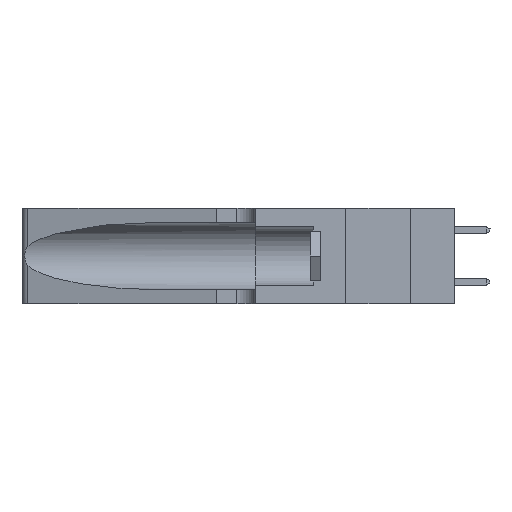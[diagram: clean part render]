
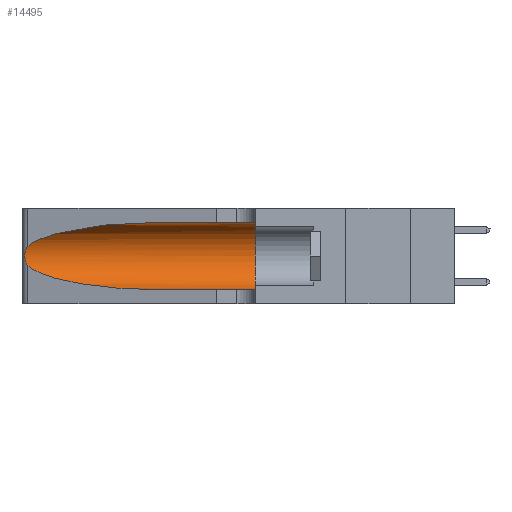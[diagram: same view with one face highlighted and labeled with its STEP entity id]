
A CAD part, left-side view. The second image highlights one B-rep face of the part: STEP entity #14495.
In plain terms, the highlighted cylindrical face has radius 3.308 mm (diameter 6.617 mm), a partial arc.
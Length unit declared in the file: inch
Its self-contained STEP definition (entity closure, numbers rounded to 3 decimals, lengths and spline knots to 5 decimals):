
#180 = ORIENTED_EDGE ( 'NONE', *, *, #1704, .T. ) ;
#356 = VERTEX_POINT ( 'NONE', #25758 ) ;
#576 = CYLINDRICAL_SURFACE ( 'NONE', #26483, 0.13025 ) ;
#1097 = CIRCLE ( 'NONE', #24617, 0.13025 ) ;
#1139 = CARTESIAN_POINT ( 'NONE',  ( 0.1305, 1.61858, 0.05475 ) ) ;
#1341 = FACE_OUTER_BOUND ( 'NONE', #19082, .T. ) ;
#1704 = EDGE_CURVE ( 'NONE', #27995, #356, #4668, .T. ) ;
#2259 = CARTESIAN_POINT ( 'NONE',  ( 0.25487, 1.22718, 0.14631 ) ) ;
#2595 = CARTESIAN_POINT ( 'NONE',  ( 0.25787, 1.23484, 0.2124 ) ) ;
#3226 = VERTEX_POINT ( 'NONE', #3661 ) ;
#3429 = ORIENTED_EDGE ( 'NONE', *, *, #3481, .F. ) ;
#3481 = EDGE_CURVE ( 'NONE', #3226, #27902, #1097, .T. ) ;
#3551 = DIRECTION ( 'NONE',  ( 0., -1., 0. ) ) ;
#3661 = CARTESIAN_POINT ( 'NONE',  ( 0.1305, 0.35, 0.31525 ) ) ;
#4051 = VERTEX_POINT ( 'NONE', #26782 ) ;
#4668 = B_SPLINE_CURVE_WITH_KNOTS ( 'NONE', 3,
 ( #29198, #12241, #17131, #2595, #19552, #5005, #22022, #7479, #24459, #9923, #26884, #12354, #29300, #14800 ),
 .UNSPECIFIED., .F., .F.,
 ( 4, 2, 2, 2, 2, 2, 4 ),
 ( 0., 0.00027, 0.00053, 0.00107, 0.0016, 0.00187, 0.00214 ),
 .UNSPECIFIED. ) ;
#5005 = CARTESIAN_POINT ( 'NONE',  ( 0.26018, 1.23835, 0.19895 ) ) ;
#6705 = CARTESIAN_POINT ( 'NONE',  ( 0.1305, 1.61858, 0.185 ) ) ;
#7057 = DIRECTION ( 'NONE',  ( 0., 1., 0. ) ) ;
#7140 = CARTESIAN_POINT ( 'NONE',  ( 0.1305, 0.72297, 0.05475 ) ) ;
#7352 = CARTESIAN_POINT ( 'NONE',  ( 0.25487, 1.22718, 0.22369 ) ) ;
#7479 = CARTESIAN_POINT ( 'NONE',  ( 0.26075, 1.23896, 0.178 ) ) ;
#7570 = CARTESIAN_POINT ( 'NONE',  ( 0.25487, 1.22718, 0.22369 ) ) ;
#7640 = EDGE_CURVE ( 'NONE', #356, #4051, #24942, .T. ) ;
#8722 = VECTOR ( 'NONE', #3551, 39.37008 ) ;
#9594 = EDGE_CURVE ( 'NONE', #25639, #27995, #13658, .T. ) ;
#9923 = CARTESIAN_POINT ( 'NONE',  ( 0.25856, 1.23593, 0.16098 ) ) ;
#11594 = DIRECTION ( 'NONE',  ( 0., 0., -1. ) ) ;
#12125 = CARTESIAN_POINT ( 'NONE',  ( 0.1305, 0.72297, 0.31525 ) ) ;
#12241 = CARTESIAN_POINT ( 'NONE',  ( 0.25555, 1.22994, 0.2215 ) ) ;
#12354 = CARTESIAN_POINT ( 'NONE',  ( 0.25639, 1.23186, 0.15144 ) ) ;
#12795 = ORIENTED_EDGE ( 'NONE', *, *, #19862, .F. ) ;
#13658 =( BOUNDED_CURVE ( )  B_SPLINE_CURVE ( 3, ( #12125, #19435, #21902, #7352 ),
 .UNSPECIFIED., .F., .F. ) 
 B_SPLINE_CURVE_WITH_KNOTS ( ( 4, 4 ),
 ( 1.5708, 2.84003 ),
 .UNSPECIFIED. ) 
 CURVE ( )  GEOMETRIC_REPRESENTATION_ITEM ( )  RATIONAL_B_SPLINE_CURVE ( ( 1., 0.87, 0.87, 1. ) ) 
 REPRESENTATION_ITEM ( '' )  );
#14286 = ORIENTED_EDGE ( 'NONE', *, *, #7640, .T. ) ;
#14410 = DIRECTION ( 'NONE',  ( 0., -1., 0. ) ) ;
#14495 = ADVANCED_FACE ( 'NONE', ( #1341 ), #576, .F. ) ;
#14800 = CARTESIAN_POINT ( 'NONE',  ( 0.25487, 1.22718, 0.14631 ) ) ;
#16094 = CARTESIAN_POINT ( 'NONE',  ( 0.1305, 0.72297, 0.31525 ) ) ;
#16589 = VECTOR ( 'NONE', #14410, 39.37008 ) ;
#17131 = CARTESIAN_POINT ( 'NONE',  ( 0.25639, 1.23184, 0.21858 ) ) ;
#19082 = EDGE_LOOP ( 'NONE', ( #22947, #180, #14286, #27629, #3429, #12795 ) ) ;
#19220 = CARTESIAN_POINT ( 'NONE',  ( 0.2373, 1.15595, 0.08982 ) ) ;
#19435 = CARTESIAN_POINT ( 'NONE',  ( 0.18966, 0.96281, 0.31525 ) ) ;
#19552 = CARTESIAN_POINT ( 'NONE',  ( 0.25854, 1.2359, 0.20912 ) ) ;
#19862 = EDGE_CURVE ( 'NONE', #25639, #3226, #23037, .T. ) ;
#21618 = CARTESIAN_POINT ( 'NONE',  ( 0.1305, 0.35, 0.185 ) ) ;
#21632 = LINE ( 'NONE', #1139, #8722 ) ;
#21636 = CARTESIAN_POINT ( 'NONE',  ( 0.1305, 1.61858, 0.31525 ) ) ;
#21693 = CARTESIAN_POINT ( 'NONE',  ( 0.18966, 0.96281, 0.05475 ) ) ;
#21902 = CARTESIAN_POINT ( 'NONE',  ( 0.2373, 1.15595, 0.28018 ) ) ;
#22022 = CARTESIAN_POINT ( 'NONE',  ( 0.26075, 1.23896, 0.19203 ) ) ;
#22947 = ORIENTED_EDGE ( 'NONE', *, *, #9594, .T. ) ;
#23037 = LINE ( 'NONE', #21636, #16589 ) ;
#23704 = DIRECTION ( 'NONE',  ( 0., -1., 0. ) ) ;
#24052 = DIRECTION ( 'NONE',  ( 0., 0., 1. ) ) ;
#24459 = CARTESIAN_POINT ( 'NONE',  ( 0.26017, 1.23833, 0.17102 ) ) ;
#24617 = AXIS2_PLACEMENT_3D ( 'NONE', #21618, #7057, #24052 ) ;
#24942 =( BOUNDED_CURVE ( )  B_SPLINE_CURVE ( 3, ( #2259, #19220, #21693, #7140 ),
 .UNSPECIFIED., .F., .F. ) 
 B_SPLINE_CURVE_WITH_KNOTS ( ( 4, 4 ),
 ( 3.44316, 4.71239 ),
 .UNSPECIFIED. ) 
 CURVE ( )  GEOMETRIC_REPRESENTATION_ITEM ( )  RATIONAL_B_SPLINE_CURVE ( ( 1., 0.87, 0.87, 1. ) ) 
 REPRESENTATION_ITEM ( '' )  );
#25639 = VERTEX_POINT ( 'NONE', #16094 ) ;
#25758 = CARTESIAN_POINT ( 'NONE',  ( 0.25487, 1.22718, 0.14631 ) ) ;
#26483 = AXIS2_PLACEMENT_3D ( 'NONE', #6705, #23704, #11594 ) ;
#26782 = CARTESIAN_POINT ( 'NONE',  ( 0.1305, 0.72297, 0.05475 ) ) ;
#26884 = CARTESIAN_POINT ( 'NONE',  ( 0.25789, 1.23486, 0.15765 ) ) ;
#27629 = ORIENTED_EDGE ( 'NONE', *, *, #30553, .T. ) ;
#27902 = VERTEX_POINT ( 'NONE', #28964 ) ;
#27995 = VERTEX_POINT ( 'NONE', #7570 ) ;
#28964 = CARTESIAN_POINT ( 'NONE',  ( 0.1305, 0.35, 0.05475 ) ) ;
#29198 = CARTESIAN_POINT ( 'NONE',  ( 0.25487, 1.22718, 0.22369 ) ) ;
#29300 = CARTESIAN_POINT ( 'NONE',  ( 0.25555, 1.22993, 0.14849 ) ) ;
#30553 = EDGE_CURVE ( 'NONE', #4051, #27902, #21632, .T. ) ;
